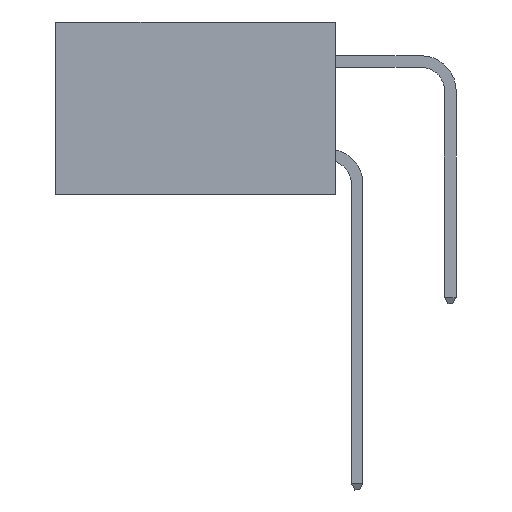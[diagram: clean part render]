
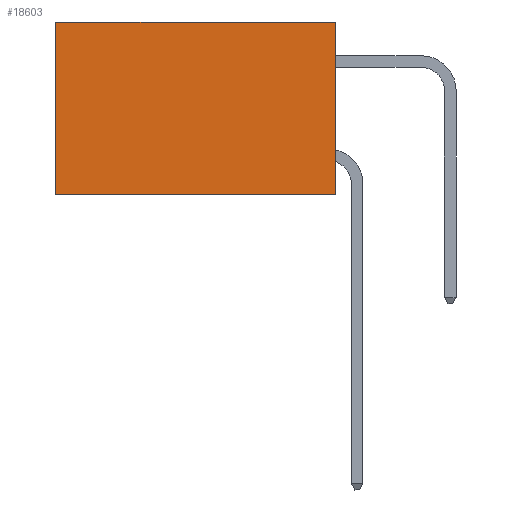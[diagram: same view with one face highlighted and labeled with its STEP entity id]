
A CAD part, left-side view. The second image highlights one B-rep face of the part: STEP entity #18603.
In plain terms, the highlighted planar face has unit normal (-1, 0, 0).
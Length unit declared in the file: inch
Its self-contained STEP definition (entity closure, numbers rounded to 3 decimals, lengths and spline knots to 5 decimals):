
#39 = DIRECTION ( 'NONE',  ( 0., 1., 0. ) ) ;
#112 = DIRECTION ( 'NONE',  ( 0., 1., 0. ) ) ;
#901 = CARTESIAN_POINT ( 'NONE',  ( 0.2875, 0.6, 0. ) ) ;
#3260 = VERTEX_POINT ( 'NONE', #37278 ) ;
#4247 = DIRECTION ( 'NONE',  ( 0., 0., -1. ) ) ;
#4850 = VERTEX_POINT ( 'NONE', #32927 ) ;
#5498 = CARTESIAN_POINT ( 'NONE',  ( 0.2875, 0., 0. ) ) ;
#6844 = CARTESIAN_POINT ( 'NONE',  ( 0.2875, 0., -0.37 ) ) ;
#7146 = LINE ( 'NONE', #5498, #17575 ) ;
#7437 = VECTOR ( 'NONE', #112, 39.37008 ) ;
#8333 = EDGE_CURVE ( 'NONE', #21590, #3260, #32647, .T. ) ;
#9526 = ORIENTED_EDGE ( 'NONE', *, *, #31450, .F. ) ;
#10229 = CARTESIAN_POINT ( 'NONE',  ( 0.2875, 0.6, -0.37 ) ) ;
#12559 = EDGE_CURVE ( 'NONE', #3260, #13109, #30790, .T. ) ;
#13109 = VERTEX_POINT ( 'NONE', #10229 ) ;
#13196 = DIRECTION ( 'NONE',  ( 1., 0., 0. ) ) ;
#15042 = AXIS2_PLACEMENT_3D ( 'NONE', #26313, #13196, #36208 ) ;
#15137 = VECTOR ( 'NONE', #39, 39.37008 ) ;
#17470 = ORIENTED_EDGE ( 'NONE', *, *, #12559, .T. ) ;
#17575 = VECTOR ( 'NONE', #41690, 39.37008 ) ;
#18524 = CARTESIAN_POINT ( 'NONE',  ( 0.2875, 0., 0. ) ) ;
#18603 = ADVANCED_FACE ( 'NONE', ( #36537 ), #42625, .F. ) ;
#21590 = VERTEX_POINT ( 'NONE', #18524 ) ;
#23073 = ORIENTED_EDGE ( 'NONE', *, *, #34313, .F. ) ;
#26313 = CARTESIAN_POINT ( 'NONE',  ( 0.2875, 0., 0. ) ) ;
#26481 = EDGE_LOOP ( 'NONE', ( #17470, #9526, #23073, #33902 ) ) ;
#30790 = LINE ( 'NONE', #901, #38468 ) ;
#31450 = EDGE_CURVE ( 'NONE', #4850, #13109, #42513, .T. ) ;
#32647 = LINE ( 'NONE', #39648, #15137 ) ;
#32927 = CARTESIAN_POINT ( 'NONE',  ( 0.2875, 0., -0.37 ) ) ;
#33902 = ORIENTED_EDGE ( 'NONE', *, *, #8333, .T. ) ;
#34313 = EDGE_CURVE ( 'NONE', #21590, #4850, #7146, .T. ) ;
#36208 = DIRECTION ( 'NONE',  ( 0., 0., -1. ) ) ;
#36537 = FACE_OUTER_BOUND ( 'NONE', #26481, .T. ) ;
#37278 = CARTESIAN_POINT ( 'NONE',  ( 0.2875, 0.6, 0. ) ) ;
#38468 = VECTOR ( 'NONE', #4247, 39.37008 ) ;
#39648 = CARTESIAN_POINT ( 'NONE',  ( 0.2875, 0., 0. ) ) ;
#41690 = DIRECTION ( 'NONE',  ( 0., 0., -1. ) ) ;
#42513 = LINE ( 'NONE', #6844, #7437 ) ;
#42625 = PLANE ( 'NONE',  #15042 ) ;
